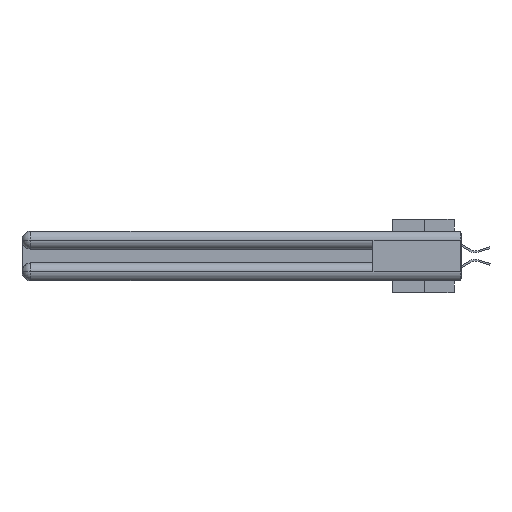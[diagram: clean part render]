
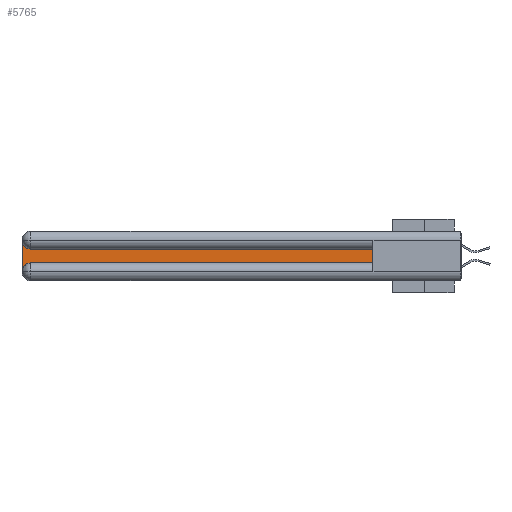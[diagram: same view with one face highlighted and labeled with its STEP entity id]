
A CAD part, left-side view. The second image highlights one B-rep face of the part: STEP entity #5765.
In plain terms, the highlighted planar face has unit normal (-1, 0, 0).
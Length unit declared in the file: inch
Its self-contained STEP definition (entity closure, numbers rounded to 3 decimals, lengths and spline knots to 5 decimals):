
#1138 = EDGE_LOOP ( 'NONE', ( #1969, #8598, #5744, #1916, #18105, #17118 ) ) ;
#1496 = CARTESIAN_POINT ( 'NONE',  ( 0.075, 0.6, -0.2175 ) ) ;
#1887 = VERTEX_POINT ( 'NONE', #22135 ) ;
#1916 = ORIENTED_EDGE ( 'NONE', *, *, #20390, .T. ) ;
#1969 = ORIENTED_EDGE ( 'NONE', *, *, #12321, .T. ) ;
#2184 = VECTOR ( 'NONE', #29934, 39.37008 ) ;
#2988 = VERTEX_POINT ( 'NONE', #24559 ) ;
#3257 = DIRECTION ( 'NONE',  ( 1., 0., 0. ) ) ;
#3788 = CARTESIAN_POINT ( 'NONE',  ( 0.075, 3., -0.2175 ) ) ;
#5355 = LINE ( 'NONE', #3788, #15019 ) ;
#5744 = ORIENTED_EDGE ( 'NONE', *, *, #21832, .T. ) ;
#5765 = ADVANCED_FACE ( 'NONE', ( #12266 ), #15627, .F. ) ;
#7535 = VERTEX_POINT ( 'NONE', #12815 ) ;
#7557 = VECTOR ( 'NONE', #20349, 39.37008 ) ;
#7749 = DIRECTION ( 'NONE',  ( 0., 0., -1. ) ) ;
#7942 = DIRECTION ( 'NONE',  ( 1., 0., 0. ) ) ;
#8533 = CARTESIAN_POINT ( 'NONE',  ( 0.075, 3., -0.1225 ) ) ;
#8598 = ORIENTED_EDGE ( 'NONE', *, *, #10293, .T. ) ;
#8600 = DIRECTION ( 'NONE',  ( 0., -1., 0. ) ) ;
#9378 = VERTEX_POINT ( 'NONE', #20103 ) ;
#10293 = EDGE_CURVE ( 'NONE', #22899, #9378, #27428, .T. ) ;
#12266 = FACE_OUTER_BOUND ( 'NONE', #1138, .T. ) ;
#12321 = EDGE_CURVE ( 'NONE', #1887, #22899, #22106, .T. ) ;
#12815 = CARTESIAN_POINT ( 'NONE',  ( 0.075, 3., -0.2775 ) ) ;
#12875 = DIRECTION ( 'NONE',  ( 0., 0., -1. ) ) ;
#13439 = EDGE_CURVE ( 'NONE', #30046, #2988, #14937, .T. ) ;
#14937 = LINE ( 'NONE', #1496, #18277 ) ;
#15019 = VECTOR ( 'NONE', #22906, 39.37008 ) ;
#15052 = CARTESIAN_POINT ( 'NONE',  ( 0.075, 2.94, -0.0625 ) ) ;
#15627 = PLANE ( 'NONE',  #20733 ) ;
#15875 = CARTESIAN_POINT ( 'NONE',  ( 0.075, 0.6, -0.1225 ) ) ;
#17118 = ORIENTED_EDGE ( 'NONE', *, *, #18015, .T. ) ;
#17211 = CARTESIAN_POINT ( 'NONE',  ( 0.075, 2.94, -0.2775 ) ) ;
#17402 = AXIS2_PLACEMENT_3D ( 'NONE', #15052, #3257, #12875 ) ;
#18015 = EDGE_CURVE ( 'NONE', #2988, #1887, #26437, .T. ) ;
#18065 = CARTESIAN_POINT ( 'NONE',  ( 0.075, 2.94, -0.2175 ) ) ;
#18105 = ORIENTED_EDGE ( 'NONE', *, *, #13439, .T. ) ;
#18277 = VECTOR ( 'NONE', #8600, 39.37008 ) ;
#19407 = AXIS2_PLACEMENT_3D ( 'NONE', #17211, #7942, #7749 ) ;
#20103 = CARTESIAN_POINT ( 'NONE',  ( 0.075, 3., -0.0625 ) ) ;
#20349 = DIRECTION ( 'NONE',  ( 0., 1., 0. ) ) ;
#20390 = EDGE_CURVE ( 'NONE', #7535, #30046, #22622, .T. ) ;
#20733 = AXIS2_PLACEMENT_3D ( 'NONE', #8533, #30130, #22836 ) ;
#21832 = EDGE_CURVE ( 'NONE', #9378, #7535, #5355, .T. ) ;
#22106 = LINE ( 'NONE', #15875, #7557 ) ;
#22135 = CARTESIAN_POINT ( 'NONE',  ( 0.075, 0.6, -0.1225 ) ) ;
#22622 = CIRCLE ( 'NONE', #19407, 0.06 ) ;
#22836 = DIRECTION ( 'NONE',  ( 0., 0., -1. ) ) ;
#22899 = VERTEX_POINT ( 'NONE', #28879 ) ;
#22906 = DIRECTION ( 'NONE',  ( 0., 0., -1. ) ) ;
#22955 = CARTESIAN_POINT ( 'NONE',  ( 0.075, 0.6, -0.2175 ) ) ;
#24559 = CARTESIAN_POINT ( 'NONE',  ( 0.075, 0.6, -0.2175 ) ) ;
#26437 = LINE ( 'NONE', #22955, #2184 ) ;
#27428 = CIRCLE ( 'NONE', #17402, 0.06 ) ;
#28879 = CARTESIAN_POINT ( 'NONE',  ( 0.075, 2.94, -0.1225 ) ) ;
#29934 = DIRECTION ( 'NONE',  ( 0., 0., 1. ) ) ;
#30046 = VERTEX_POINT ( 'NONE', #18065 ) ;
#30130 = DIRECTION ( 'NONE',  ( 1., 0., 0. ) ) ;
